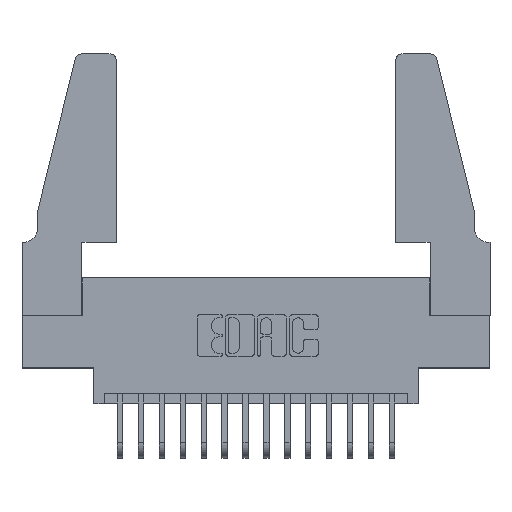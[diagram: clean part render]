
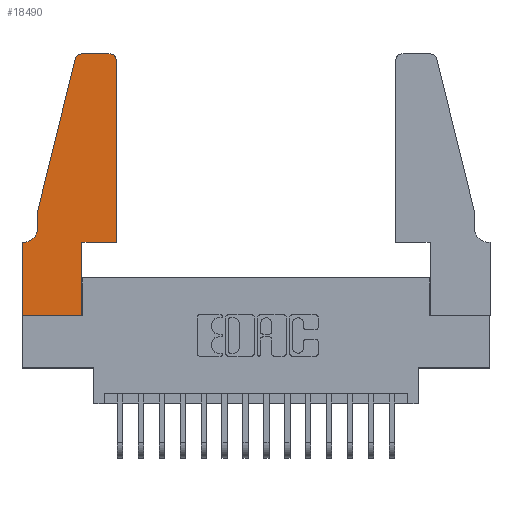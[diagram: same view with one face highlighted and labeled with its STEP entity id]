
A CAD part, top view. The second image highlights one B-rep face of the part: STEP entity #18490.
In plain terms, the highlighted planar face has unit normal (0, 0, 1).
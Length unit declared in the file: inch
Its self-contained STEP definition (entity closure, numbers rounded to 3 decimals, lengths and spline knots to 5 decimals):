
#518 = VERTEX_POINT ( 'NONE', #5657 ) ;
#579 = DIRECTION ( 'NONE',  ( 0., 0., 1. ) ) ;
#602 = ORIENTED_EDGE ( 'NONE', *, *, #1457, .T. ) ;
#802 = AXIS2_PLACEMENT_3D ( 'NONE', #6202, #16187, #7646 ) ;
#1144 = EDGE_LOOP ( 'NONE', ( #17787, #3593, #8756, #7389, #2965, #602, #15507, #8700, #2779, #5481, #10627, #11840 ) ) ;
#1263 = LINE ( 'NONE', #13912, #12354 ) ;
#1342 = EDGE_CURVE ( 'NONE', #518, #4686, #14583, .T. ) ;
#1370 = EDGE_CURVE ( 'NONE', #8426, #3878, #14151, .T. ) ;
#1457 = EDGE_CURVE ( 'NONE', #15597, #12391, #1263, .T. ) ;
#1481 = CARTESIAN_POINT ( 'NONE',  ( 0.0055, 0.35, 0.37 ) ) ;
#1531 = VECTOR ( 'NONE', #12999, 39.37008 ) ;
#1615 = CARTESIAN_POINT ( 'NONE',  ( 0.4505, 0.35, 0.37 ) ) ;
#1657 = VERTEX_POINT ( 'NONE', #11587 ) ;
#2137 = CARTESIAN_POINT ( 'NONE',  ( 0., 0., 0.37 ) ) ;
#2374 = CIRCLE ( 'NONE', #802, 0.03 ) ;
#2779 = ORIENTED_EDGE ( 'NONE', *, *, #17563, .T. ) ;
#2965 = ORIENTED_EDGE ( 'NONE', *, *, #7446, .T. ) ;
#3223 = VECTOR ( 'NONE', #16367, 39.37008 ) ;
#3480 = DIRECTION ( 'NONE',  ( 0., 0., 1. ) ) ;
#3593 = ORIENTED_EDGE ( 'NONE', *, *, #4031, .T. ) ;
#3810 = CARTESIAN_POINT ( 'NONE',  ( 0., 0., 0.37 ) ) ;
#3878 = VERTEX_POINT ( 'NONE', #17395 ) ;
#3882 = EDGE_CURVE ( 'NONE', #3878, #6884, #9606, .T. ) ;
#4031 = EDGE_CURVE ( 'NONE', #13047, #518, #18281, .T. ) ;
#4483 = CIRCLE ( 'NONE', #17651, 0.07 ) ;
#4686 = VERTEX_POINT ( 'NONE', #6391 ) ;
#5481 = ORIENTED_EDGE ( 'NONE', *, *, #1370, .T. ) ;
#5498 = VECTOR ( 'NONE', #17322, 39.37008 ) ;
#5657 = CARTESIAN_POINT ( 'NONE',  ( 0.25487, 1.22718, 0.37 ) ) ;
#5696 = DIRECTION ( 'NONE',  ( -0.239, -0.971, 0. ) ) ;
#5778 = VECTOR ( 'NONE', #14618, 39.37008 ) ;
#5915 = EDGE_CURVE ( 'NONE', #1657, #18324, #11085, .T. ) ;
#5942 = LINE ( 'NONE', #18693, #5498 ) ;
#6072 = VECTOR ( 'NONE', #6588, 39.37008 ) ;
#6202 = CARTESIAN_POINT ( 'NONE',  ( 0.4205, 1.22, 0.37 ) ) ;
#6391 = CARTESIAN_POINT ( 'NONE',  ( 0.0755, 0.5, 0.37 ) ) ;
#6521 = CARTESIAN_POINT ( 'NONE',  ( 0.0055, 0.42, 0.37 ) ) ;
#6588 = DIRECTION ( 'NONE',  ( 1., 0., 0. ) ) ;
#6680 = AXIS2_PLACEMENT_3D ( 'NONE', #17840, #579, #10764 ) ;
#6719 = CARTESIAN_POINT ( 'NONE',  ( 0.4505, 0.35, 0.37 ) ) ;
#6884 = VERTEX_POINT ( 'NONE', #8095 ) ;
#7213 = VERTEX_POINT ( 'NONE', #10296 ) ;
#7287 = VECTOR ( 'NONE', #16528, 39.37008 ) ;
#7389 = ORIENTED_EDGE ( 'NONE', *, *, #17946, .T. ) ;
#7446 = EDGE_CURVE ( 'NONE', #7213, #15597, #4483, .T. ) ;
#7646 = DIRECTION ( 'NONE',  ( 1., 0., 0. ) ) ;
#7862 = PLANE ( 'NONE',  #6680 ) ;
#7951 = DIRECTION ( 'NONE',  ( -1., 0., 0. ) ) ;
#8095 = CARTESIAN_POINT ( 'NONE',  ( 0.4505, 1.22, 0.37 ) ) ;
#8426 = VERTEX_POINT ( 'NONE', #8680 ) ;
#8680 = CARTESIAN_POINT ( 'NONE',  ( 0.2865, 0.35, 0.37 ) ) ;
#8700 = ORIENTED_EDGE ( 'NONE', *, *, #5915, .T. ) ;
#8756 = ORIENTED_EDGE ( 'NONE', *, *, #1342, .T. ) ;
#9606 = LINE ( 'NONE', #1615, #5778 ) ;
#9792 = DIRECTION ( 'NONE',  ( -1., 0., 0. ) ) ;
#9847 = EDGE_CURVE ( 'NONE', #12391, #1657, #18574, .T. ) ;
#10089 = CARTESIAN_POINT ( 'NONE',  ( 0.2865, 0., 0.37 ) ) ;
#10296 = CARTESIAN_POINT ( 'NONE',  ( 0.0755, 0.42, 0.37 ) ) ;
#10627 = ORIENTED_EDGE ( 'NONE', *, *, #3882, .T. ) ;
#10764 = DIRECTION ( 'NONE',  ( 1., 0., 0. ) ) ;
#10821 = EDGE_CURVE ( 'NONE', #6884, #15034, #2374, .T. ) ;
#11085 = LINE ( 'NONE', #2137, #7287 ) ;
#11554 = CARTESIAN_POINT ( 'NONE',  ( 0.2605, 1.25, 0.37 ) ) ;
#11587 = CARTESIAN_POINT ( 'NONE',  ( 0., 0., 0.37 ) ) ;
#11840 = ORIENTED_EDGE ( 'NONE', *, *, #10821, .T. ) ;
#11871 = CARTESIAN_POINT ( 'NONE',  ( 0., 0.35, 0.37 ) ) ;
#12079 = CARTESIAN_POINT ( 'NONE',  ( 0.0755, 0.5, 0.37 ) ) ;
#12115 = CARTESIAN_POINT ( 'NONE',  ( 0.284, 1.22, 0.37 ) ) ;
#12354 = VECTOR ( 'NONE', #9792, 39.37008 ) ;
#12391 = VERTEX_POINT ( 'NONE', #11871 ) ;
#12437 = DIRECTION ( 'NONE',  ( 0., -1., 0. ) ) ;
#12474 = CARTESIAN_POINT ( 'NONE',  ( 0.0755, 0.5, 0.37 ) ) ;
#12631 = LINE ( 'NONE', #11554, #1531 ) ;
#12999 = DIRECTION ( 'NONE',  ( -1., 0., 0. ) ) ;
#13047 = VERTEX_POINT ( 'NONE', #16131 ) ;
#13165 = AXIS2_PLACEMENT_3D ( 'NONE', #12115, #3480, #13552 ) ;
#13552 = DIRECTION ( 'NONE',  ( 1., 0., 0. ) ) ;
#13912 = CARTESIAN_POINT ( 'NONE',  ( 0.0755, 0.35, 0.37 ) ) ;
#14151 = LINE ( 'NONE', #6719, #6072 ) ;
#14210 = EDGE_CURVE ( 'NONE', #15034, #13047, #12631, .T. ) ;
#14253 = LINE ( 'NONE', #12079, #3223 ) ;
#14583 = LINE ( 'NONE', #12474, #18362 ) ;
#14618 = DIRECTION ( 'NONE',  ( 0., 1., 0. ) ) ;
#14627 = CARTESIAN_POINT ( 'NONE',  ( 0.4205, 1.25, 0.37 ) ) ;
#15034 = VERTEX_POINT ( 'NONE', #14627 ) ;
#15242 = VECTOR ( 'NONE', #12437, 39.37008 ) ;
#15507 = ORIENTED_EDGE ( 'NONE', *, *, #9847, .T. ) ;
#15597 = VERTEX_POINT ( 'NONE', #1481 ) ;
#15780 = FACE_OUTER_BOUND ( 'NONE', #1144, .T. ) ;
#16131 = CARTESIAN_POINT ( 'NONE',  ( 0.284, 1.25, 0.37 ) ) ;
#16187 = DIRECTION ( 'NONE',  ( 0., 0., 1. ) ) ;
#16367 = DIRECTION ( 'NONE',  ( 0., -1., 0. ) ) ;
#16506 = DIRECTION ( 'NONE',  ( 0., 0., -1. ) ) ;
#16528 = DIRECTION ( 'NONE',  ( 1., 0., 0. ) ) ;
#17322 = DIRECTION ( 'NONE',  ( 0., 1., 0. ) ) ;
#17395 = CARTESIAN_POINT ( 'NONE',  ( 0.4505, 0.35, 0.37 ) ) ;
#17563 = EDGE_CURVE ( 'NONE', #18324, #8426, #5942, .T. ) ;
#17651 = AXIS2_PLACEMENT_3D ( 'NONE', #6521, #16506, #7951 ) ;
#17787 = ORIENTED_EDGE ( 'NONE', *, *, #14210, .T. ) ;
#17840 = CARTESIAN_POINT ( 'NONE',  ( 0., 0.35, 0.37 ) ) ;
#17946 = EDGE_CURVE ( 'NONE', #4686, #7213, #14253, .T. ) ;
#18281 = CIRCLE ( 'NONE', #13165, 0.03 ) ;
#18324 = VERTEX_POINT ( 'NONE', #10089 ) ;
#18362 = VECTOR ( 'NONE', #5696, 39.37008 ) ;
#18490 = ADVANCED_FACE ( 'NONE', ( #15780 ), #7862, .T. ) ;
#18574 = LINE ( 'NONE', #3810, #15242 ) ;
#18693 = CARTESIAN_POINT ( 'NONE',  ( 0.2865, 0.35, 0.37 ) ) ;
